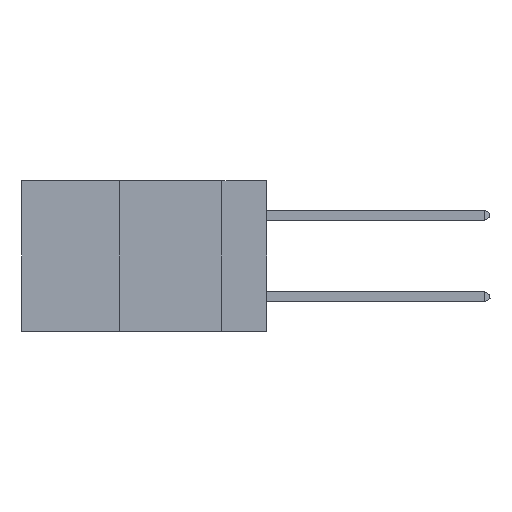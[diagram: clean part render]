
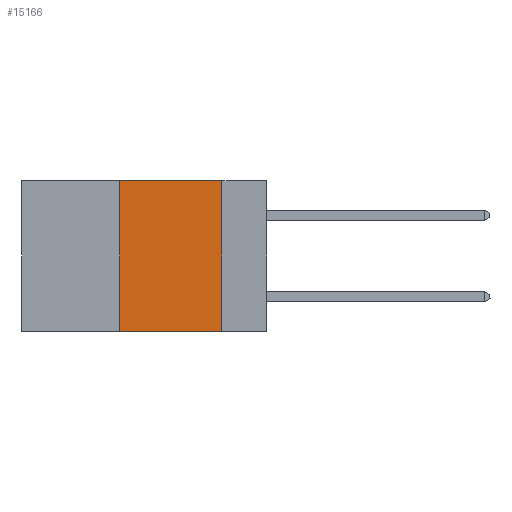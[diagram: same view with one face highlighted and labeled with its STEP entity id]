
A CAD part, left-side view. The second image highlights one B-rep face of the part: STEP entity #15166.
In plain terms, the highlighted planar face has unit normal (-1, 0, 0).
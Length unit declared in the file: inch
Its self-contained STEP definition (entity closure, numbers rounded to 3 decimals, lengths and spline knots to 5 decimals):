
#367 = DIRECTION ( 'NONE',  ( 1., 0., 0. ) ) ;
#379 = AXIS2_PLACEMENT_3D ( 'NONE', #8334, #367, #1964 ) ;
#487 = ORIENTED_EDGE ( 'NONE', *, *, #20172, .F. ) ;
#604 = VERTEX_POINT ( 'NONE', #19742 ) ;
#965 = ORIENTED_EDGE ( 'NONE', *, *, #2687, .F. ) ;
#976 = CARTESIAN_POINT ( 'NONE',  ( 0., 0.11, 0. ) ) ;
#1579 = VECTOR ( 'NONE', #13195, 39.37008 ) ;
#1964 = DIRECTION ( 'NONE',  ( 0., 0., -1. ) ) ;
#2260 = CARTESIAN_POINT ( 'NONE',  ( 0., 0.6, 0. ) ) ;
#2687 = EDGE_CURVE ( 'NONE', #4880, #8083, #20760, .T. ) ;
#4880 = VERTEX_POINT ( 'NONE', #16856 ) ;
#5002 = EDGE_CURVE ( 'NONE', #604, #4880, #16876, .T. ) ;
#6272 = FACE_OUTER_BOUND ( 'NONE', #19883, .T. ) ;
#7927 = ORIENTED_EDGE ( 'NONE', *, *, #8482, .T. ) ;
#8078 = CARTESIAN_POINT ( 'NONE',  ( 0., 0.11, -0.37 ) ) ;
#8083 = VERTEX_POINT ( 'NONE', #976 ) ;
#8334 = CARTESIAN_POINT ( 'NONE',  ( 0., 0.6, 0. ) ) ;
#8482 = EDGE_CURVE ( 'NONE', #604, #19345, #13213, .T. ) ;
#13195 = DIRECTION ( 'NONE',  ( 0., 0., -1. ) ) ;
#13213 = LINE ( 'NONE', #13800, #17497 ) ;
#13216 = VECTOR ( 'NONE', #16713, 39.37008 ) ;
#13800 = CARTESIAN_POINT ( 'NONE',  ( 0., 0.6, -0.37 ) ) ;
#14647 = PLANE ( 'NONE',  #379 ) ;
#14720 = CARTESIAN_POINT ( 'NONE',  ( 0., 0.36, 0. ) ) ;
#14896 = LINE ( 'NONE', #19474, #1579 ) ;
#15166 = ADVANCED_FACE ( 'NONE', ( #6272 ), #14647, .F. ) ;
#15571 = DIRECTION ( 'NONE',  ( 0., 0., 1. ) ) ;
#16713 = DIRECTION ( 'NONE',  ( 0., -1., 0. ) ) ;
#16856 = CARTESIAN_POINT ( 'NONE',  ( 0., 0.36, 0. ) ) ;
#16876 = LINE ( 'NONE', #14720, #18133 ) ;
#17343 = ORIENTED_EDGE ( 'NONE', *, *, #5002, .F. ) ;
#17497 = VECTOR ( 'NONE', #18758, 39.37008 ) ;
#18133 = VECTOR ( 'NONE', #15571, 39.37008 ) ;
#18758 = DIRECTION ( 'NONE',  ( 0., -1., 0. ) ) ;
#19345 = VERTEX_POINT ( 'NONE', #8078 ) ;
#19474 = CARTESIAN_POINT ( 'NONE',  ( 0., 0.11, 0. ) ) ;
#19742 = CARTESIAN_POINT ( 'NONE',  ( 0., 0.36, -0.37 ) ) ;
#19883 = EDGE_LOOP ( 'NONE', ( #487, #965, #17343, #7927 ) ) ;
#20172 = EDGE_CURVE ( 'NONE', #8083, #19345, #14896, .T. ) ;
#20760 = LINE ( 'NONE', #2260, #13216 ) ;
